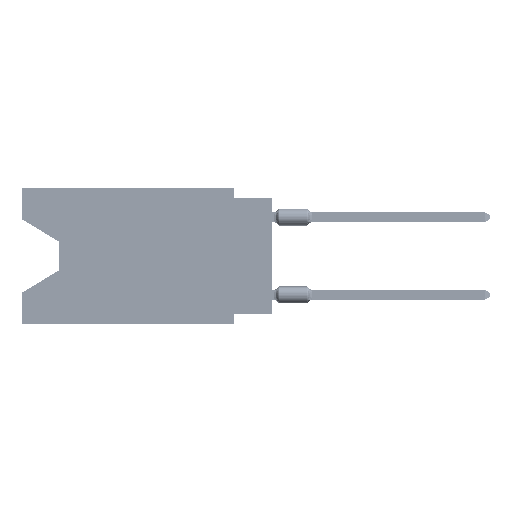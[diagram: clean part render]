
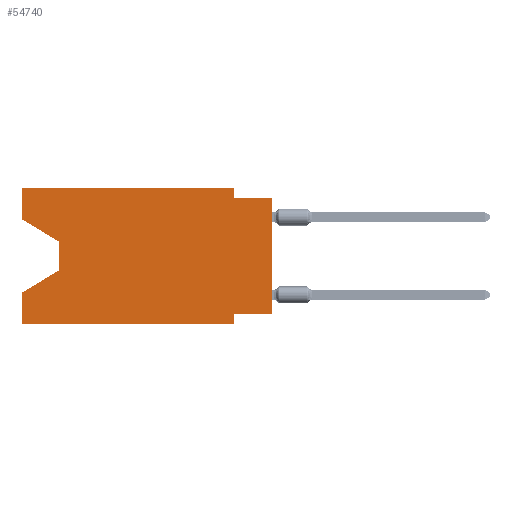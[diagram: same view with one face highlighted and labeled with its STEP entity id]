
A CAD part, left-side view. The second image highlights one B-rep face of the part: STEP entity #54740.
In plain terms, the highlighted planar face has unit normal (-1, 0, 0).
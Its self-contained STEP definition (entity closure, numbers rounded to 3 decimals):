
#1533 = VECTOR ( 'NONE', #4745, 1000. ) ;
#1907 = DIRECTION ( 'NONE',  ( 0., 0., -1. ) ) ;
#4745 = DIRECTION ( 'NONE',  ( 0., 0.855, -0.519 ) ) ;
#4795 = EDGE_CURVE ( 'NONE', #16804, #19504, #75959, .T. ) ;
#5865 = LINE ( 'NONE', #41237, #10603 ) ;
#6823 = CARTESIAN_POINT ( 'NONE',  ( 0., 16.383, 0. ) ) ;
#7103 = VECTOR ( 'NONE', #77349, 1000. ) ;
#7411 = DIRECTION ( 'NONE',  ( 0., 0., 1. ) ) ;
#8860 = VECTOR ( 'NONE', #32858, 1000. ) ;
#9222 = CARTESIAN_POINT ( 'NONE',  ( 0., 0., -0.635 ) ) ;
#10603 = VECTOR ( 'NONE', #33896, 1000. ) ;
#12573 = CARTESIAN_POINT ( 'NONE',  ( 0., 16.383, 0. ) ) ;
#13196 = VERTEX_POINT ( 'NONE', #86810 ) ;
#14995 = CARTESIAN_POINT ( 'NONE',  ( 0., 13.97, -5.385 ) ) ;
#16279 = EDGE_CURVE ( 'NONE', #74475, #44297, #90251, .T. ) ;
#16804 = VERTEX_POINT ( 'NONE', #71183 ) ;
#17817 = DIRECTION ( 'NONE',  ( 0., 0., -1. ) ) ;
#18082 = LINE ( 'NONE', #74616, #73030 ) ;
#18265 = CARTESIAN_POINT ( 'NONE',  ( 0., 13.97, -3.505 ) ) ;
#18588 = LINE ( 'NONE', #23699, #49414 ) ;
#19504 = VERTEX_POINT ( 'NONE', #9222 ) ;
#22497 = LINE ( 'NONE', #79458, #37201 ) ;
#23170 = ORIENTED_EDGE ( 'NONE', *, *, #88516, .T. ) ;
#23362 = EDGE_CURVE ( 'NONE', #13196, #19504, #18588, .T. ) ;
#23480 = ORIENTED_EDGE ( 'NONE', *, *, #71628, .F. ) ;
#23699 = CARTESIAN_POINT ( 'NONE',  ( 0., 0., 0. ) ) ;
#24966 = ORIENTED_EDGE ( 'NONE', *, *, #80496, .F. ) ;
#25627 = VERTEX_POINT ( 'NONE', #14995 ) ;
#26377 = ORIENTED_EDGE ( 'NONE', *, *, #85149, .T. ) ;
#26444 = ORIENTED_EDGE ( 'NONE', *, *, #23362, .T. ) ;
#26515 = VECTOR ( 'NONE', #66522, 1000. ) ;
#30388 = ORIENTED_EDGE ( 'NONE', *, *, #43297, .T. ) ;
#30981 = VERTEX_POINT ( 'NONE', #70936 ) ;
#32858 = DIRECTION ( 'NONE',  ( 0., 0., 1. ) ) ;
#32896 = DIRECTION ( 'NONE',  ( 0., -0.855, -0.519 ) ) ;
#33510 = DIRECTION ( 'NONE',  ( 0., -1., 0. ) ) ;
#33896 = DIRECTION ( 'NONE',  ( 0., 1., 0. ) ) ;
#37201 = VECTOR ( 'NONE', #50045, 1000. ) ;
#37223 = AXIS2_PLACEMENT_3D ( 'NONE', #73440, #53175, #17817 ) ;
#37293 = CARTESIAN_POINT ( 'NONE',  ( 0., 2.54, -8.89 ) ) ;
#37978 = EDGE_CURVE ( 'NONE', #48474, #30981, #76672, .T. ) ;
#38343 = VERTEX_POINT ( 'NONE', #39398 ) ;
#38348 = CARTESIAN_POINT ( 'NONE',  ( 0., 16.383, -6.852 ) ) ;
#39398 = CARTESIAN_POINT ( 'NONE',  ( 0., 2.54, -8.255 ) ) ;
#40085 = EDGE_CURVE ( 'NONE', #68120, #48255, #60025, .T. ) ;
#40600 = LINE ( 'NONE', #12573, #7103 ) ;
#40981 = ORIENTED_EDGE ( 'NONE', *, *, #51808, .F. ) ;
#41115 = CARTESIAN_POINT ( 'NONE',  ( 0., 16.383, 0. ) ) ;
#41237 = CARTESIAN_POINT ( 'NONE',  ( 0., 0., -8.255 ) ) ;
#42464 = ORIENTED_EDGE ( 'NONE', *, *, #74190, .F. ) ;
#43297 = EDGE_CURVE ( 'NONE', #25627, #44297, #67263, .T. ) ;
#44297 = VERTEX_POINT ( 'NONE', #38348 ) ;
#45837 = VERTEX_POINT ( 'NONE', #73630 ) ;
#46901 = CARTESIAN_POINT ( 'NONE',  ( 0., 16.383, 0. ) ) ;
#48255 = VERTEX_POINT ( 'NONE', #85990 ) ;
#48474 = VERTEX_POINT ( 'NONE', #46901 ) ;
#49414 = VECTOR ( 'NONE', #7411, 1000. ) ;
#50045 = DIRECTION ( 'NONE',  ( 0., -1., 0. ) ) ;
#51808 = EDGE_CURVE ( 'NONE', #13196, #38343, #5865, .T. ) ;
#52448 = LINE ( 'NONE', #37293, #77720 ) ;
#53175 = DIRECTION ( 'NONE',  ( 1., 0., 0. ) ) ;
#54351 = ORIENTED_EDGE ( 'NONE', *, *, #16279, .F. ) ;
#54740 = ADVANCED_FACE ( 'NONE', ( #81214 ), #74324, .F. ) ;
#59179 = LINE ( 'NONE', #18265, #26515 ) ;
#60025 = LINE ( 'NONE', #80263, #64534 ) ;
#62652 = VECTOR ( 'NONE', #75048, 1000. ) ;
#63993 = CARTESIAN_POINT ( 'NONE',  ( 0., 16.383, -2.038 ) ) ;
#64135 = VECTOR ( 'NONE', #33510, 1000. ) ;
#64534 = VECTOR ( 'NONE', #32896, 1000. ) ;
#66522 = DIRECTION ( 'NONE',  ( 0., 0., -1. ) ) ;
#67263 = LINE ( 'NONE', #67709, #1533 ) ;
#67709 = CARTESIAN_POINT ( 'NONE',  ( 0., 13.97, -5.385 ) ) ;
#67716 = DIRECTION ( 'NONE',  ( 0., 0., -1. ) ) ;
#68120 = VERTEX_POINT ( 'NONE', #63993 ) ;
#70936 = CARTESIAN_POINT ( 'NONE',  ( 0., 2.54, 0. ) ) ;
#71183 = CARTESIAN_POINT ( 'NONE',  ( 0., 2.54, -0.635 ) ) ;
#71628 = EDGE_CURVE ( 'NONE', #30981, #16804, #18082, .T. ) ;
#73030 = VECTOR ( 'NONE', #67716, 1000. ) ;
#73440 = CARTESIAN_POINT ( 'NONE',  ( 0., 16.383, 0. ) ) ;
#73552 = ORIENTED_EDGE ( 'NONE', *, *, #37978, .F. ) ;
#73630 = CARTESIAN_POINT ( 'NONE',  ( 0., 2.54, -8.89 ) ) ;
#74190 = EDGE_CURVE ( 'NONE', #38343, #45837, #52448, .T. ) ;
#74324 = PLANE ( 'NONE',  #37223 ) ;
#74475 = VERTEX_POINT ( 'NONE', #74939 ) ;
#74616 = CARTESIAN_POINT ( 'NONE',  ( 0., 2.54, 0. ) ) ;
#74939 = CARTESIAN_POINT ( 'NONE',  ( 0., 16.383, -8.89 ) ) ;
#75048 = DIRECTION ( 'NONE',  ( 0., -1., 0. ) ) ;
#75959 = LINE ( 'NONE', #89280, #62652 ) ;
#76672 = LINE ( 'NONE', #6823, #64135 ) ;
#77349 = DIRECTION ( 'NONE',  ( 0., 0., 1. ) ) ;
#77720 = VECTOR ( 'NONE', #1907, 1000. ) ;
#79458 = CARTESIAN_POINT ( 'NONE',  ( 0., 16.383, -8.89 ) ) ;
#80263 = CARTESIAN_POINT ( 'NONE',  ( 0., 16.383, -2.038 ) ) ;
#80275 = ORIENTED_EDGE ( 'NONE', *, *, #40085, .T. ) ;
#80496 = EDGE_CURVE ( 'NONE', #68120, #48474, #40600, .T. ) ;
#81214 = FACE_OUTER_BOUND ( 'NONE', #87761, .T. ) ;
#83471 = ORIENTED_EDGE ( 'NONE', *, *, #4795, .F. ) ;
#85149 = EDGE_CURVE ( 'NONE', #48255, #25627, #59179, .T. ) ;
#85990 = CARTESIAN_POINT ( 'NONE',  ( 0., 13.97, -3.505 ) ) ;
#86810 = CARTESIAN_POINT ( 'NONE',  ( 0., 0., -8.255 ) ) ;
#87761 = EDGE_LOOP ( 'NONE', ( #80275, #26377, #30388, #54351, #23170, #42464, #40981, #26444, #83471, #23480, #73552, #24966 ) ) ;
#88516 = EDGE_CURVE ( 'NONE', #74475, #45837, #22497, .T. ) ;
#89280 = CARTESIAN_POINT ( 'NONE',  ( 0., 0., -0.635 ) ) ;
#90251 = LINE ( 'NONE', #41115, #8860 ) ;
